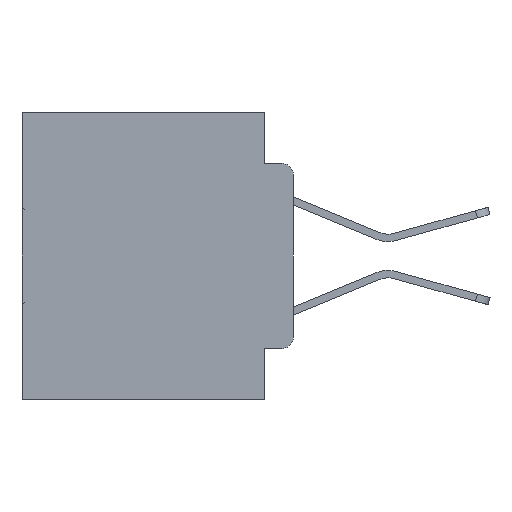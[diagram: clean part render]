
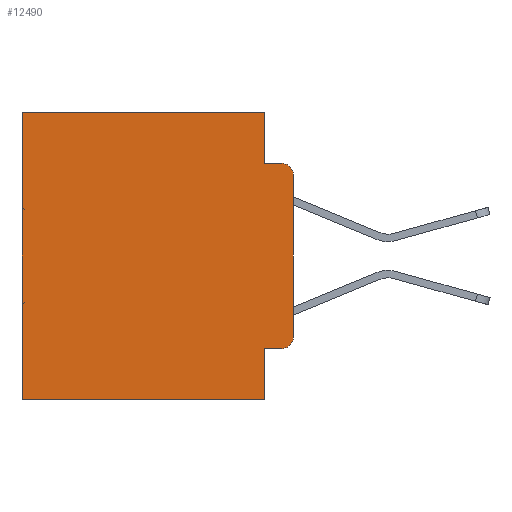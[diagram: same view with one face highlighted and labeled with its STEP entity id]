
A CAD part, left-side view. The second image highlights one B-rep face of the part: STEP entity #12490.
In plain terms, the highlighted planar face has unit normal (-1, 0, 0).
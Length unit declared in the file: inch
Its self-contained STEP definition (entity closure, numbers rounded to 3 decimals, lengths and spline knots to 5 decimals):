
#435 = CARTESIAN_POINT ( 'NONE',  ( 0.298, 0.473, -0.5 ) ) ;
#953 = VECTOR ( 'NONE', #2102, 39.37008 ) ;
#1166 = CARTESIAN_POINT ( 'NONE',  ( 0.298, 0., -0.3915 ) ) ;
#1377 = DIRECTION ( 'NONE',  ( -1., 0., 0. ) ) ;
#1960 = EDGE_CURVE ( 'NONE', #16091, #17786, #29905, .T. ) ;
#2102 = DIRECTION ( 'NONE',  ( 0., 1., 0. ) ) ;
#2513 = LINE ( 'NONE', #8116, #24434 ) ;
#2861 = EDGE_LOOP ( 'NONE', ( #11189, #27480, #3159, #23235, #8390, #17158, #9578, #4712, #18776, #32170 ) ) ;
#3083 = AXIS2_PLACEMENT_3D ( 'NONE', #11448, #3711, #22079 ) ;
#3159 = ORIENTED_EDGE ( 'NONE', *, *, #11416, .F. ) ;
#3711 = DIRECTION ( 'NONE',  ( 1., 0., 0. ) ) ;
#4712 = ORIENTED_EDGE ( 'NONE', *, *, #19982, .F. ) ;
#4730 = DIRECTION ( 'NONE',  ( 0., 0., -1. ) ) ;
#5423 = DIRECTION ( 'NONE',  ( 0., 0., -1. ) ) ;
#5736 = FACE_OUTER_BOUND ( 'NONE', #2861, .T. ) ;
#5766 = EDGE_CURVE ( 'NONE', #23219, #21467, #9976, .T. ) ;
#6724 = LINE ( 'NONE', #20075, #19926 ) ;
#7178 = CARTESIAN_POINT ( 'NONE',  ( 0.298, 0.02, -0.4115 ) ) ;
#7678 = EDGE_CURVE ( 'NONE', #23219, #33132, #2513, .T. ) ;
#8116 = CARTESIAN_POINT ( 'NONE',  ( 0.298, 0., 0. ) ) ;
#8390 = ORIENTED_EDGE ( 'NONE', *, *, #1960, .T. ) ;
#8873 = PLANE ( 'NONE',  #3083 ) ;
#9000 = CARTESIAN_POINT ( 'NONE',  ( 0.298, 0.051, 0. ) ) ;
#9578 = ORIENTED_EDGE ( 'NONE', *, *, #25208, .F. ) ;
#9976 = CIRCLE ( 'NONE', #31007, 0.02 ) ;
#11189 = ORIENTED_EDGE ( 'NONE', *, *, #7678, .F. ) ;
#11351 = CARTESIAN_POINT ( 'NONE',  ( 0.298, 0.051, -0.0885 ) ) ;
#11416 = EDGE_CURVE ( 'NONE', #22731, #21467, #19172, .T. ) ;
#11448 = CARTESIAN_POINT ( 'NONE',  ( 0.298, 0., 0. ) ) ;
#12490 = ADVANCED_FACE ( 'NONE', ( #5736 ), #8873, .F. ) ;
#12831 = CARTESIAN_POINT ( 'NONE',  ( 0.298, 0., -0.5 ) ) ;
#15086 = VECTOR ( 'NONE', #28807, 39.37008 ) ;
#15253 = CARTESIAN_POINT ( 'NONE',  ( 0.298, 0.051, -0.4115 ) ) ;
#15560 = CARTESIAN_POINT ( 'NONE',  ( 0.298, 0.02, -0.0885 ) ) ;
#16091 = VERTEX_POINT ( 'NONE', #9000 ) ;
#16349 = VERTEX_POINT ( 'NONE', #16913 ) ;
#16913 = CARTESIAN_POINT ( 'NONE',  ( 0.298, 0.051, -0.4115 ) ) ;
#17068 = CARTESIAN_POINT ( 'NONE',  ( 0.298, 0.02, -0.3915 ) ) ;
#17071 = LINE ( 'NONE', #15253, #20786 ) ;
#17092 = VERTEX_POINT ( 'NONE', #28701 ) ;
#17158 = ORIENTED_EDGE ( 'NONE', *, *, #25891, .T. ) ;
#17700 = LINE ( 'NONE', #32273, #29645 ) ;
#17786 = VERTEX_POINT ( 'NONE', #18019 ) ;
#17881 = DIRECTION ( 'NONE',  ( -1., 0., 0. ) ) ;
#18019 = CARTESIAN_POINT ( 'NONE',  ( 0.298, 0.473, 0. ) ) ;
#18776 = ORIENTED_EDGE ( 'NONE', *, *, #25305, .T. ) ;
#19172 = LINE ( 'NONE', #31229, #15086 ) ;
#19926 = VECTOR ( 'NONE', #28059, 39.37008 ) ;
#19982 = EDGE_CURVE ( 'NONE', #16349, #17092, #17700, .T. ) ;
#20075 = CARTESIAN_POINT ( 'NONE',  ( 0.298, 0.473, 0. ) ) ;
#20550 = VERTEX_POINT ( 'NONE', #7178 ) ;
#20786 = VECTOR ( 'NONE', #33650, 39.37008 ) ;
#21216 = DIRECTION ( 'NONE',  ( 0., 1., 0. ) ) ;
#21410 = DIRECTION ( 'NONE',  ( 0., 0., -1. ) ) ;
#21467 = VERTEX_POINT ( 'NONE', #15560 ) ;
#22079 = DIRECTION ( 'NONE',  ( 0., 0., -1. ) ) ;
#22638 = DIRECTION ( 'NONE',  ( 0., 0., -1. ) ) ;
#22705 = LINE ( 'NONE', #23778, #30100 ) ;
#22731 = VERTEX_POINT ( 'NONE', #11351 ) ;
#23219 = VERTEX_POINT ( 'NONE', #23817 ) ;
#23235 = ORIENTED_EDGE ( 'NONE', *, *, #27654, .F. ) ;
#23352 = CARTESIAN_POINT ( 'NONE',  ( 0.298, 0.02, -0.1085 ) ) ;
#23778 = CARTESIAN_POINT ( 'NONE',  ( 0.298, 0.051, 0. ) ) ;
#23817 = CARTESIAN_POINT ( 'NONE',  ( 0.298, 0., -0.1085 ) ) ;
#24434 = VECTOR ( 'NONE', #21410, 39.37008 ) ;
#25208 = EDGE_CURVE ( 'NONE', #17092, #29794, #29428, .T. ) ;
#25305 = EDGE_CURVE ( 'NONE', #16349, #20550, #17071, .T. ) ;
#25891 = EDGE_CURVE ( 'NONE', #17786, #29794, #6724, .T. ) ;
#27480 = ORIENTED_EDGE ( 'NONE', *, *, #5766, .T. ) ;
#27654 = EDGE_CURVE ( 'NONE', #16091, #22731, #22705, .T. ) ;
#28059 = DIRECTION ( 'NONE',  ( 0., 0., -1. ) ) ;
#28633 = DIRECTION ( 'NONE',  ( 0., 0., -1. ) ) ;
#28701 = CARTESIAN_POINT ( 'NONE',  ( 0.298, 0.051, -0.5 ) ) ;
#28807 = DIRECTION ( 'NONE',  ( 0., -1., 0. ) ) ;
#29428 = LINE ( 'NONE', #12831, #953 ) ;
#29645 = VECTOR ( 'NONE', #5423, 39.37008 ) ;
#29794 = VERTEX_POINT ( 'NONE', #435 ) ;
#29905 = LINE ( 'NONE', #31673, #32351 ) ;
#29962 = EDGE_CURVE ( 'NONE', #20550, #33132, #30381, .T. ) ;
#30100 = VECTOR ( 'NONE', #28633, 39.37008 ) ;
#30107 = AXIS2_PLACEMENT_3D ( 'NONE', #17068, #1377, #22638 ) ;
#30381 = CIRCLE ( 'NONE', #30107, 0.02 ) ;
#31007 = AXIS2_PLACEMENT_3D ( 'NONE', #23352, #17881, #4730 ) ;
#31229 = CARTESIAN_POINT ( 'NONE',  ( 0.298, 0.051, -0.0885 ) ) ;
#31673 = CARTESIAN_POINT ( 'NONE',  ( 0.298, 0., 0. ) ) ;
#32170 = ORIENTED_EDGE ( 'NONE', *, *, #29962, .T. ) ;
#32273 = CARTESIAN_POINT ( 'NONE',  ( 0.298, 0.051, 0. ) ) ;
#32351 = VECTOR ( 'NONE', #21216, 39.37008 ) ;
#33132 = VERTEX_POINT ( 'NONE', #1166 ) ;
#33650 = DIRECTION ( 'NONE',  ( 0., -1., 0. ) ) ;
